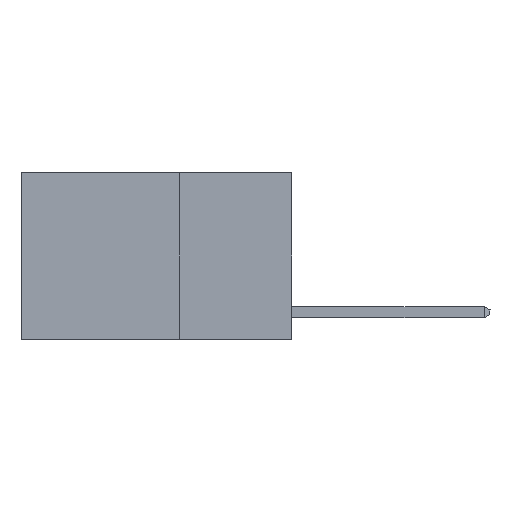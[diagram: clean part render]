
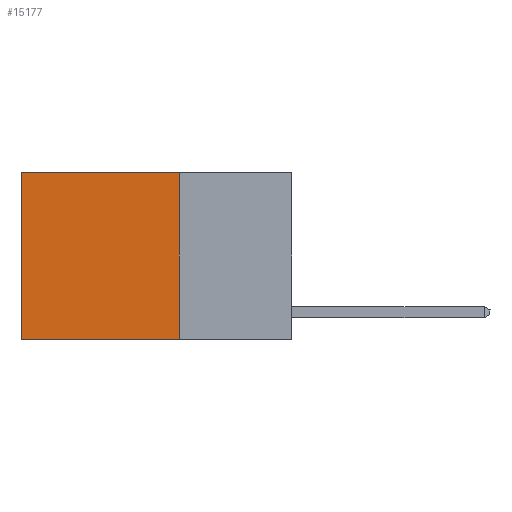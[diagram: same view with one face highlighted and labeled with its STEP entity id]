
A CAD part, left-side view. The second image highlights one B-rep face of the part: STEP entity #15177.
In plain terms, the highlighted planar face has unit normal (-1, 0, 0).
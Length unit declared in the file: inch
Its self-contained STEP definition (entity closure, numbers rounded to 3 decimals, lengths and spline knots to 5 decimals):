
#121 = ORIENTED_EDGE ( 'NONE', *, *, #11150, .F. ) ;
#959 = CARTESIAN_POINT ( 'NONE',  ( 0.2625, 0.6, -0.37 ) ) ;
#1627 = VERTEX_POINT ( 'NONE', #16160 ) ;
#2703 = PLANE ( 'NONE',  #15450 ) ;
#4392 = EDGE_LOOP ( 'NONE', ( #16773, #16609, #121, #13877 ) ) ;
#4471 = DIRECTION ( 'NONE',  ( 0., 0., -1. ) ) ;
#5315 = FACE_OUTER_BOUND ( 'NONE', #4392, .T. ) ;
#5606 = CARTESIAN_POINT ( 'NONE',  ( 0.2625, 0.25, -0.37 ) ) ;
#5652 = LINE ( 'NONE', #14946, #14375 ) ;
#6063 = VECTOR ( 'NONE', #6528, 39.37008 ) ;
#6155 = DIRECTION ( 'NONE',  ( 0., 1., 0. ) ) ;
#6191 = DIRECTION ( 'NONE',  ( 1., 0., 0. ) ) ;
#6528 = DIRECTION ( 'NONE',  ( 0., 0., -1. ) ) ;
#8455 = CARTESIAN_POINT ( 'NONE',  ( 0.2625, 0.6, 0. ) ) ;
#9061 = CARTESIAN_POINT ( 'NONE',  ( 0.2625, 0.25, 0. ) ) ;
#10933 = VERTEX_POINT ( 'NONE', #9061 ) ;
#11150 = EDGE_CURVE ( 'NONE', #10933, #1627, #5652, .T. ) ;
#13783 = VECTOR ( 'NONE', #17841, 39.37008 ) ;
#13877 = ORIENTED_EDGE ( 'NONE', *, *, #17451, .T. ) ;
#14375 = VECTOR ( 'NONE', #4471, 39.37008 ) ;
#14946 = CARTESIAN_POINT ( 'NONE',  ( 0.2625, 0.25, 0. ) ) ;
#15177 = ADVANCED_FACE ( 'NONE', ( #5315 ), #2703, .F. ) ;
#15450 = AXIS2_PLACEMENT_3D ( 'NONE', #16676, #6191, #18435 ) ;
#16160 = CARTESIAN_POINT ( 'NONE',  ( 0.2625, 0.25, -0.37 ) ) ;
#16609 = ORIENTED_EDGE ( 'NONE', *, *, #20041, .F. ) ;
#16676 = CARTESIAN_POINT ( 'NONE',  ( 0.2625, 0.25, 0. ) ) ;
#16773 = ORIENTED_EDGE ( 'NONE', *, *, #21627, .T. ) ;
#17451 = EDGE_CURVE ( 'NONE', #10933, #21122, #20008, .T. ) ;
#17841 = DIRECTION ( 'NONE',  ( 0., 1., 0. ) ) ;
#17911 = LINE ( 'NONE', #5606, #13783 ) ;
#18435 = DIRECTION ( 'NONE',  ( 0., 0., -1. ) ) ;
#18781 = CARTESIAN_POINT ( 'NONE',  ( 0.2625, 0.6, 0. ) ) ;
#19447 = VECTOR ( 'NONE', #6155, 39.37008 ) ;
#20008 = LINE ( 'NONE', #21864, #19447 ) ;
#20041 = EDGE_CURVE ( 'NONE', #1627, #21466, #17911, .T. ) ;
#20056 = LINE ( 'NONE', #18781, #6063 ) ;
#21122 = VERTEX_POINT ( 'NONE', #8455 ) ;
#21466 = VERTEX_POINT ( 'NONE', #959 ) ;
#21627 = EDGE_CURVE ( 'NONE', #21122, #21466, #20056, .T. ) ;
#21864 = CARTESIAN_POINT ( 'NONE',  ( 0.2625, 0.25, 0. ) ) ;
